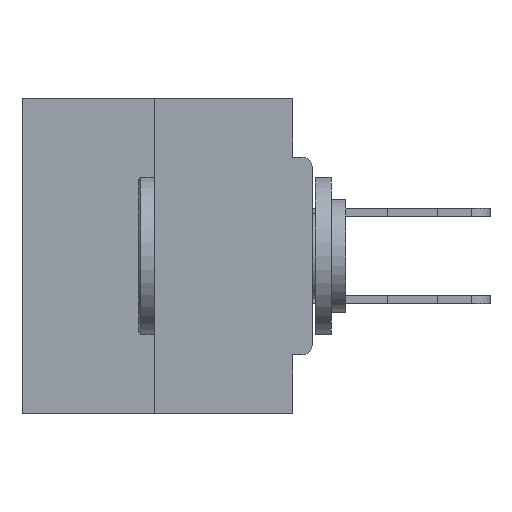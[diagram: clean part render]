
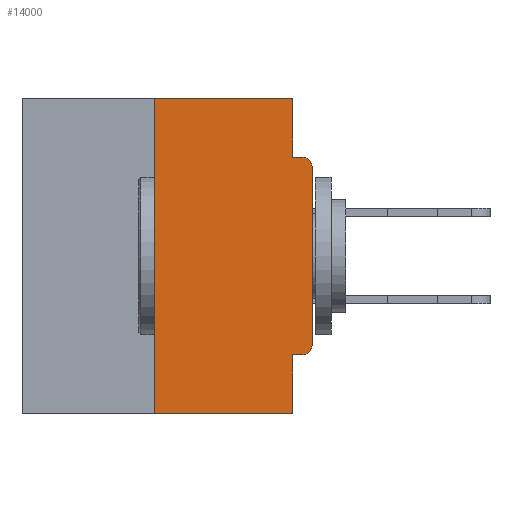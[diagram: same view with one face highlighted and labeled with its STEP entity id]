
A CAD part, left-side view. The second image highlights one B-rep face of the part: STEP entity #14000.
In plain terms, the highlighted planar face has unit normal (-1, 0, 0).
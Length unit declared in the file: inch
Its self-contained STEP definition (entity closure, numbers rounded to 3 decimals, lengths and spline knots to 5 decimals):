
#597 = EDGE_CURVE ( 'NONE', #18998, #28579, #29947, .T. ) ;
#733 = VECTOR ( 'NONE', #19675, 39.37008 ) ;
#767 = AXIS2_PLACEMENT_3D ( 'NONE', #3081, #19326, #24896 ) ;
#1052 = EDGE_CURVE ( 'NONE', #31054, #20342, #16433, .T. ) ;
#1071 = EDGE_LOOP ( 'NONE', ( #10621, #18733, #3401, #19588, #13770, #21762, #33843, #22589, #21629, #17252 ) ) ;
#1539 = CIRCLE ( 'NONE', #29512, 0.015 ) ;
#1691 = FACE_OUTER_BOUND ( 'NONE', #1071, .T. ) ;
#3081 = CARTESIAN_POINT ( 'NONE',  ( 0., 0.46, 0. ) ) ;
#3201 = VECTOR ( 'NONE', #6900, 39.37008 ) ;
#3401 = ORIENTED_EDGE ( 'NONE', *, *, #7625, .T. ) ;
#4140 = CARTESIAN_POINT ( 'NONE',  ( 0., 0.031, 0. ) ) ;
#4157 = VERTEX_POINT ( 'NONE', #32333 ) ;
#6565 = DIRECTION ( 'NONE',  ( -1., 0., 0. ) ) ;
#6729 = VERTEX_POINT ( 'NONE', #11076 ) ;
#6900 = DIRECTION ( 'NONE',  ( 0., 0., 1. ) ) ;
#7625 = EDGE_CURVE ( 'NONE', #4157, #33908, #8191, .T. ) ;
#7982 = CARTESIAN_POINT ( 'NONE',  ( 0., 0., -0.0935 ) ) ;
#8191 = LINE ( 'NONE', #12449, #22946 ) ;
#8646 = EDGE_CURVE ( 'NONE', #20342, #18998, #16803, .T. ) ;
#8716 = VECTOR ( 'NONE', #31192, 39.37008 ) ;
#9275 = CARTESIAN_POINT ( 'NONE',  ( 0., 0., -0.1085 ) ) ;
#10562 = LINE ( 'NONE', #29008, #3201 ) ;
#10621 = ORIENTED_EDGE ( 'NONE', *, *, #1052, .F. ) ;
#10799 = VERTEX_POINT ( 'NONE', #23030 ) ;
#11076 = CARTESIAN_POINT ( 'NONE',  ( 0., 0.015, -0.4065 ) ) ;
#11160 = DIRECTION ( 'NONE',  ( -1., 0., 0. ) ) ;
#11279 = CARTESIAN_POINT ( 'NONE',  ( 0., 0.015, -0.1085 ) ) ;
#12149 = CARTESIAN_POINT ( 'NONE',  ( 0., 0.031, -0.0935 ) ) ;
#12449 = CARTESIAN_POINT ( 'NONE',  ( 0., 0.46, -0.5 ) ) ;
#12656 = CARTESIAN_POINT ( 'NONE',  ( 0., 0.031, -0.4065 ) ) ;
#13313 = CARTESIAN_POINT ( 'NONE',  ( 0., 0., -0.4065 ) ) ;
#13387 = CARTESIAN_POINT ( 'NONE',  ( 0., 0.46, 0. ) ) ;
#13770 = ORIENTED_EDGE ( 'NONE', *, *, #29456, .F. ) ;
#13943 = DIRECTION ( 'NONE',  ( 0., 0., -1. ) ) ;
#14000 = ADVANCED_FACE ( 'NONE', ( #1691 ), #30400, .F. ) ;
#14702 = VECTOR ( 'NONE', #26992, 39.37008 ) ;
#15186 = VECTOR ( 'NONE', #19361, 39.37008 ) ;
#16433 = LINE ( 'NONE', #13387, #14702 ) ;
#16803 = LINE ( 'NONE', #25815, #32456 ) ;
#17050 = CARTESIAN_POINT ( 'NONE',  ( 0., 0.015, -0.0935 ) ) ;
#17252 = ORIENTED_EDGE ( 'NONE', *, *, #8646, .F. ) ;
#17633 = LINE ( 'NONE', #35638, #733 ) ;
#18192 = LINE ( 'NONE', #22917, #8716 ) ;
#18733 = ORIENTED_EDGE ( 'NONE', *, *, #21561, .F. ) ;
#18998 = VERTEX_POINT ( 'NONE', #12149 ) ;
#19326 = DIRECTION ( 'NONE',  ( 1., 0., 0. ) ) ;
#19361 = DIRECTION ( 'NONE',  ( 0., -1., 0. ) ) ;
#19588 = ORIENTED_EDGE ( 'NONE', *, *, #23863, .F. ) ;
#19675 = DIRECTION ( 'NONE',  ( 0., 0., 1. ) ) ;
#19754 = VERTEX_POINT ( 'NONE', #9275 ) ;
#19955 = CIRCLE ( 'NONE', #19986, 0.015 ) ;
#19986 = AXIS2_PLACEMENT_3D ( 'NONE', #11279, #11160, #13943 ) ;
#20342 = VERTEX_POINT ( 'NONE', #4140 ) ;
#21561 = EDGE_CURVE ( 'NONE', #4157, #31054, #10562, .T. ) ;
#21629 = ORIENTED_EDGE ( 'NONE', *, *, #597, .F. ) ;
#21762 = ORIENTED_EDGE ( 'NONE', *, *, #31117, .T. ) ;
#22589 = ORIENTED_EDGE ( 'NONE', *, *, #32120, .T. ) ;
#22805 = CARTESIAN_POINT ( 'NONE',  ( 0., 0.015, -0.3915 ) ) ;
#22917 = CARTESIAN_POINT ( 'NONE',  ( 0., 0.031, -0.5 ) ) ;
#22946 = VECTOR ( 'NONE', #26385, 39.37008 ) ;
#23030 = CARTESIAN_POINT ( 'NONE',  ( 0., 0., -0.3915 ) ) ;
#23775 = VECTOR ( 'NONE', #35328, 39.37008 ) ;
#23863 = EDGE_CURVE ( 'NONE', #31222, #33908, #18192, .T. ) ;
#24896 = DIRECTION ( 'NONE',  ( 0., 0., -1. ) ) ;
#25815 = CARTESIAN_POINT ( 'NONE',  ( 0., 0.031, 0. ) ) ;
#25950 = DIRECTION ( 'NONE',  ( 0., 0., -1. ) ) ;
#26385 = DIRECTION ( 'NONE',  ( 0., -1., 0. ) ) ;
#26992 = DIRECTION ( 'NONE',  ( 0., -1., 0. ) ) ;
#28425 = CARTESIAN_POINT ( 'NONE',  ( 0., 0.25, 0. ) ) ;
#28579 = VERTEX_POINT ( 'NONE', #17050 ) ;
#29008 = CARTESIAN_POINT ( 'NONE',  ( 0., 0.25, 0. ) ) ;
#29456 = EDGE_CURVE ( 'NONE', #6729, #31222, #33387, .T. ) ;
#29512 = AXIS2_PLACEMENT_3D ( 'NONE', #22805, #6565, #25950 ) ;
#29947 = LINE ( 'NONE', #7982, #15186 ) ;
#30400 = PLANE ( 'NONE',  #767 ) ;
#30705 = CARTESIAN_POINT ( 'NONE',  ( 0., 0.031, -0.5 ) ) ;
#31054 = VERTEX_POINT ( 'NONE', #28425 ) ;
#31117 = EDGE_CURVE ( 'NONE', #6729, #10799, #1539, .T. ) ;
#31192 = DIRECTION ( 'NONE',  ( 0., 0., -1. ) ) ;
#31222 = VERTEX_POINT ( 'NONE', #12656 ) ;
#31922 = DIRECTION ( 'NONE',  ( 0., 0., -1. ) ) ;
#32120 = EDGE_CURVE ( 'NONE', #19754, #28579, #19955, .T. ) ;
#32333 = CARTESIAN_POINT ( 'NONE',  ( 0., 0.25, -0.5 ) ) ;
#32456 = VECTOR ( 'NONE', #31922, 39.37008 ) ;
#33387 = LINE ( 'NONE', #13313, #23775 ) ;
#33843 = ORIENTED_EDGE ( 'NONE', *, *, #34948, .T. ) ;
#33908 = VERTEX_POINT ( 'NONE', #30705 ) ;
#34948 = EDGE_CURVE ( 'NONE', #10799, #19754, #17633, .T. ) ;
#35328 = DIRECTION ( 'NONE',  ( 0., 1., 0. ) ) ;
#35638 = CARTESIAN_POINT ( 'NONE',  ( 0., 0., 0. ) ) ;
